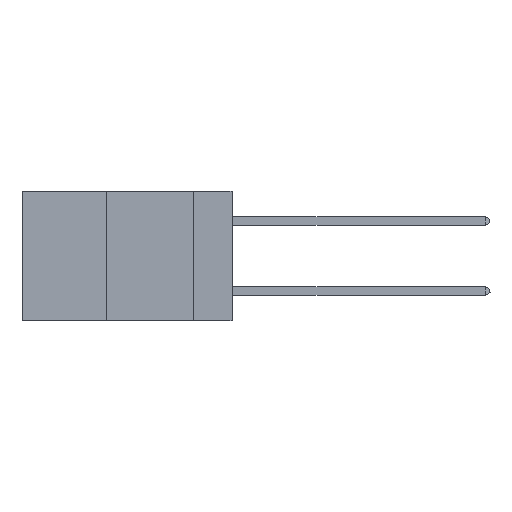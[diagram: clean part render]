
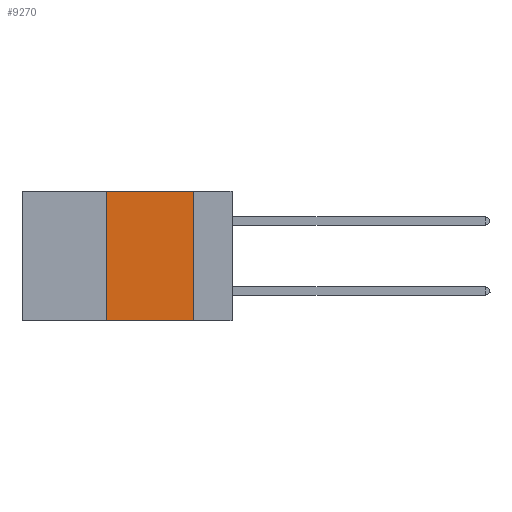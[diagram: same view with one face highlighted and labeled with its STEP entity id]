
A CAD part, left-side view. The second image highlights one B-rep face of the part: STEP entity #9270.
In plain terms, the highlighted planar face has unit normal (-1, 0, 0).
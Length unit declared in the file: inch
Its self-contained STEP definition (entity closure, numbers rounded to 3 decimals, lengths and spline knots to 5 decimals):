
#170 = CARTESIAN_POINT ( 'NONE',  ( 0., 0.11, 0. ) ) ;
#5057 = CARTESIAN_POINT ( 'NONE',  ( 0., 0.6, 0. ) ) ;
#5279 = VECTOR ( 'NONE', #7411, 39.37008 ) ;
#5386 = AXIS2_PLACEMENT_3D ( 'NONE', #11871, #14185, #14287 ) ;
#6598 = ORIENTED_EDGE ( 'NONE', *, *, #28545, .F. ) ;
#7120 = EDGE_LOOP ( 'NONE', ( #6598, #10700, #9577, #7663 ) ) ;
#7411 = DIRECTION ( 'NONE',  ( 0., -1., 0. ) ) ;
#7663 = ORIENTED_EDGE ( 'NONE', *, *, #10311, .T. ) ;
#9270 = ADVANCED_FACE ( 'NONE', ( #11429 ), #16688, .F. ) ;
#9577 = ORIENTED_EDGE ( 'NONE', *, *, #17201, .F. ) ;
#10105 = LINE ( 'NONE', #10154, #16973 ) ;
#10154 = CARTESIAN_POINT ( 'NONE',  ( 0., 0.36, 0. ) ) ;
#10311 = EDGE_CURVE ( 'NONE', #26251, #16577, #26152, .T. ) ;
#10700 = ORIENTED_EDGE ( 'NONE', *, *, #19020, .F. ) ;
#11429 = FACE_OUTER_BOUND ( 'NONE', #7120, .T. ) ;
#11435 = VERTEX_POINT ( 'NONE', #15547 ) ;
#11871 = CARTESIAN_POINT ( 'NONE',  ( 0., 0.6, 0. ) ) ;
#14185 = DIRECTION ( 'NONE',  ( 1., 0., 0. ) ) ;
#14287 = DIRECTION ( 'NONE',  ( 0., 0., -1. ) ) ;
#14770 = VECTOR ( 'NONE', #18538, 39.37008 ) ;
#15547 = CARTESIAN_POINT ( 'NONE',  ( 0., 0.36, 0. ) ) ;
#15772 = LINE ( 'NONE', #17380, #26893 ) ;
#16577 = VERTEX_POINT ( 'NONE', #21071 ) ;
#16688 = PLANE ( 'NONE',  #5386 ) ;
#16973 = VECTOR ( 'NONE', #21535, 39.37008 ) ;
#17201 = EDGE_CURVE ( 'NONE', #26251, #11435, #10105, .T. ) ;
#17380 = CARTESIAN_POINT ( 'NONE',  ( 0., 0.11, 0. ) ) ;
#18007 = LINE ( 'NONE', #5057, #14770 ) ;
#18538 = DIRECTION ( 'NONE',  ( 0., -1., 0. ) ) ;
#19003 = CARTESIAN_POINT ( 'NONE',  ( 0., 0.6, -0.37 ) ) ;
#19020 = EDGE_CURVE ( 'NONE', #11435, #29627, #18007, .T. ) ;
#21071 = CARTESIAN_POINT ( 'NONE',  ( 0., 0.11, -0.37 ) ) ;
#21535 = DIRECTION ( 'NONE',  ( 0., 0., 1. ) ) ;
#22189 = DIRECTION ( 'NONE',  ( 0., 0., -1. ) ) ;
#23132 = CARTESIAN_POINT ( 'NONE',  ( 0., 0.36, -0.37 ) ) ;
#26152 = LINE ( 'NONE', #19003, #5279 ) ;
#26251 = VERTEX_POINT ( 'NONE', #23132 ) ;
#26893 = VECTOR ( 'NONE', #22189, 39.37008 ) ;
#28545 = EDGE_CURVE ( 'NONE', #29627, #16577, #15772, .T. ) ;
#29627 = VERTEX_POINT ( 'NONE', #170 ) ;
